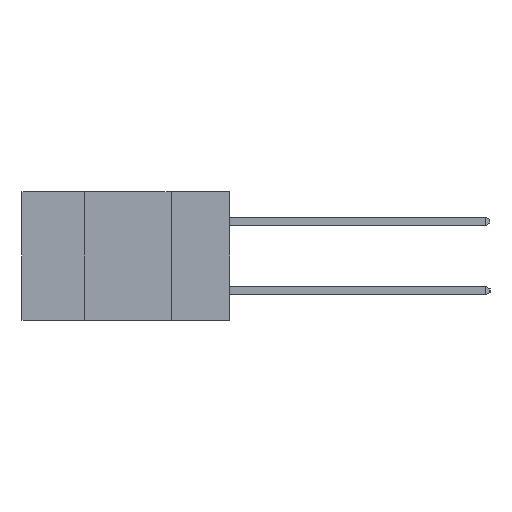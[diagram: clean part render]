
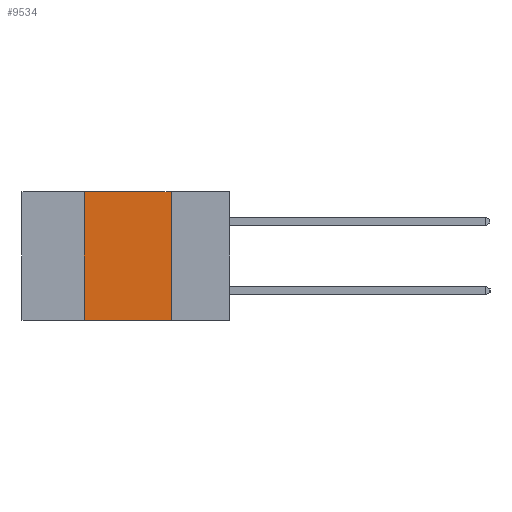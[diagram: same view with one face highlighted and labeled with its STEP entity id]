
A CAD part, left-side view. The second image highlights one B-rep face of the part: STEP entity #9534.
In plain terms, the highlighted planar face has unit normal (-1, 0, 0).
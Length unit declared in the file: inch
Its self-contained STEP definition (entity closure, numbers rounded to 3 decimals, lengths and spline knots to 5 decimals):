
#59 = CARTESIAN_POINT ( 'NONE',  ( 0., 0.42, -0.37 ) ) ;
#892 = VECTOR ( 'NONE', #8223, 39.37008 ) ;
#1122 = DIRECTION ( 'NONE',  ( 0., 0., -1. ) ) ;
#1371 = LINE ( 'NONE', #7821, #892 ) ;
#1971 = VECTOR ( 'NONE', #3322, 39.37008 ) ;
#2036 = FACE_OUTER_BOUND ( 'NONE', #4436, .T. ) ;
#2103 = LINE ( 'NONE', #7865, #1971 ) ;
#2722 = ORIENTED_EDGE ( 'NONE', *, *, #5654, .F. ) ;
#2947 = VERTEX_POINT ( 'NONE', #7488 ) ;
#3164 = EDGE_CURVE ( 'NONE', #3857, #5516, #1371, .T. ) ;
#3322 = DIRECTION ( 'NONE',  ( 0., -1., 0. ) ) ;
#3340 = CARTESIAN_POINT ( 'NONE',  ( 0., 0.17, 0. ) ) ;
#3440 = DIRECTION ( 'NONE',  ( 0., 0., -1. ) ) ;
#3691 = VECTOR ( 'NONE', #1122, 39.37008 ) ;
#3857 = VERTEX_POINT ( 'NONE', #9081 ) ;
#3913 = LINE ( 'NONE', #6312, #3691 ) ;
#4207 = ORIENTED_EDGE ( 'NONE', *, *, #5934, .F. ) ;
#4273 = VECTOR ( 'NONE', #8029, 39.37008 ) ;
#4436 = EDGE_LOOP ( 'NONE', ( #5960, #4207, #2722, #8298 ) ) ;
#5204 = AXIS2_PLACEMENT_3D ( 'NONE', #9471, #7990, #3440 ) ;
#5516 = VERTEX_POINT ( 'NONE', #7929 ) ;
#5616 = VERTEX_POINT ( 'NONE', #3340 ) ;
#5654 = EDGE_CURVE ( 'NONE', #3857, #2947, #6272, .T. ) ;
#5934 = EDGE_CURVE ( 'NONE', #2947, #5616, #2103, .T. ) ;
#5949 = EDGE_CURVE ( 'NONE', #5616, #5516, #3913, .T. ) ;
#5960 = ORIENTED_EDGE ( 'NONE', *, *, #5949, .F. ) ;
#6272 = LINE ( 'NONE', #59, #4273 ) ;
#6312 = CARTESIAN_POINT ( 'NONE',  ( 0., 0.17, -0.37 ) ) ;
#6404 = PLANE ( 'NONE',  #5204 ) ;
#7488 = CARTESIAN_POINT ( 'NONE',  ( 0., 0.42, 0. ) ) ;
#7821 = CARTESIAN_POINT ( 'NONE',  ( 0., 0.6, -0.37 ) ) ;
#7865 = CARTESIAN_POINT ( 'NONE',  ( 0., 0.6, 0. ) ) ;
#7929 = CARTESIAN_POINT ( 'NONE',  ( 0., 0.17, -0.37 ) ) ;
#7990 = DIRECTION ( 'NONE',  ( 1., 0., 0. ) ) ;
#8029 = DIRECTION ( 'NONE',  ( 0., 0., 1. ) ) ;
#8223 = DIRECTION ( 'NONE',  ( 0., -1., 0. ) ) ;
#8298 = ORIENTED_EDGE ( 'NONE', *, *, #3164, .T. ) ;
#9081 = CARTESIAN_POINT ( 'NONE',  ( 0., 0.42, -0.37 ) ) ;
#9471 = CARTESIAN_POINT ( 'NONE',  ( 0., 0.6, 0. ) ) ;
#9534 = ADVANCED_FACE ( 'NONE', ( #2036 ), #6404, .F. ) ;
